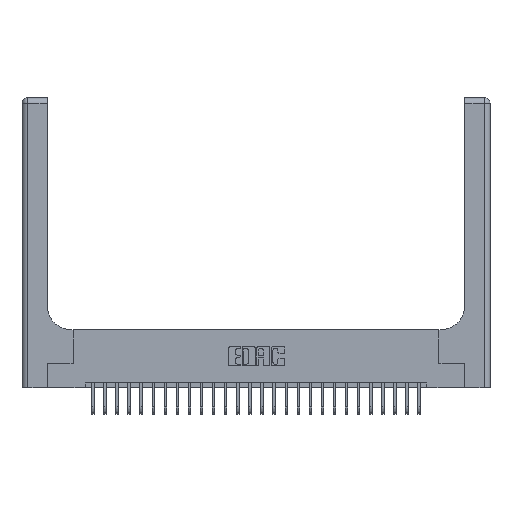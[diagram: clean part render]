
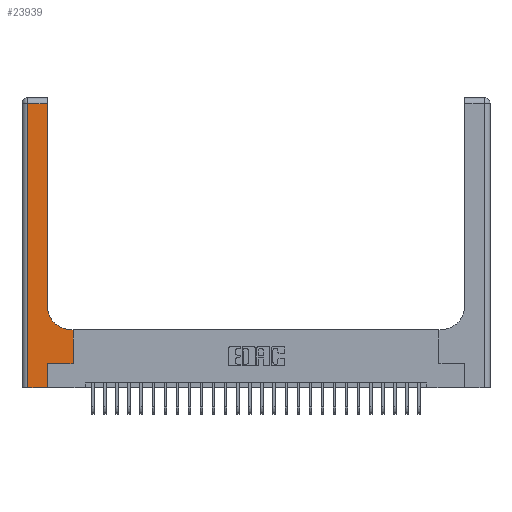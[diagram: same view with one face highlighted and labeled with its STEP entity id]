
A CAD part, top view. The second image highlights one B-rep face of the part: STEP entity #23939.
In plain terms, the highlighted planar face has unit normal (0, 0, 1).
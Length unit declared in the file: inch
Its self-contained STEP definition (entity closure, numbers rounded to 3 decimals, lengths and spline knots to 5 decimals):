
#5 = ORIENTED_EDGE ( 'NONE', *, *, #5332, .T. ) ;
#142 = DIRECTION ( 'NONE',  ( -1., 0., 0. ) ) ;
#563 = CARTESIAN_POINT ( 'NONE',  ( 0.528, 0.25, 0.37 ) ) ;
#609 = VECTOR ( 'NONE', #4721, 39.37008 ) ;
#1825 = CARTESIAN_POINT ( 'NONE',  ( 0.51, 0.6, 0.37 ) ) ;
#2618 = DIRECTION ( 'NONE',  ( 0., 0., -1. ) ) ;
#2772 = DIRECTION ( 'NONE',  ( 0., -1., 0. ) ) ;
#3071 = CIRCLE ( 'NONE', #6296, 0.25 ) ;
#3143 = VERTEX_POINT ( 'NONE', #11806 ) ;
#3183 = AXIS2_PLACEMENT_3D ( 'NONE', #24445, #14598, #14859 ) ;
#3644 = EDGE_LOOP ( 'NONE', ( #12751, #5, #16306, #23933, #14509, #15662, #12771, #17433, #15202 ) ) ;
#4266 = VERTEX_POINT ( 'NONE', #15007 ) ;
#4280 = LINE ( 'NONE', #23768, #8020 ) ;
#4721 = DIRECTION ( 'NONE',  ( -1., 0., 0. ) ) ;
#4760 = DIRECTION ( 'NONE',  ( 1., 0., 0. ) ) ;
#5100 = FACE_OUTER_BOUND ( 'NONE', #3644, .T. ) ;
#5332 = EDGE_CURVE ( 'NONE', #16618, #10583, #10309, .T. ) ;
#5795 = CARTESIAN_POINT ( 'NONE',  ( 0.06, 0., 0.37 ) ) ;
#5812 = CARTESIAN_POINT ( 'NONE',  ( 0.26, 0.6, 0.37 ) ) ;
#5923 = VECTOR ( 'NONE', #142, 39.37008 ) ;
#6296 = AXIS2_PLACEMENT_3D ( 'NONE', #23634, #2618, #4760 ) ;
#6320 = LINE ( 'NONE', #6701, #24600 ) ;
#6701 = CARTESIAN_POINT ( 'NONE',  ( 0.06, 3., 0.37 ) ) ;
#7499 = EDGE_CURVE ( 'NONE', #19654, #24125, #23149, .T. ) ;
#7681 = VECTOR ( 'NONE', #22227, 39.37008 ) ;
#8020 = VECTOR ( 'NONE', #18230, 39.37008 ) ;
#8192 = CARTESIAN_POINT ( 'NONE',  ( 0.26, 2.94, 0.37 ) ) ;
#9288 = PLANE ( 'NONE',  #3183 ) ;
#9572 = EDGE_CURVE ( 'NONE', #4266, #11926, #24064, .T. ) ;
#9664 = VECTOR ( 'NONE', #15995, 39.37008 ) ;
#10309 = LINE ( 'NONE', #23840, #609 ) ;
#10583 = VERTEX_POINT ( 'NONE', #20242 ) ;
#11655 = EDGE_CURVE ( 'NONE', #20416, #16618, #4280, .T. ) ;
#11806 = CARTESIAN_POINT ( 'NONE',  ( 0.528, 0.25, 0.37 ) ) ;
#11926 = VERTEX_POINT ( 'NONE', #19480 ) ;
#12156 = CARTESIAN_POINT ( 'NONE',  ( 0.265, 0.25, 0.37 ) ) ;
#12219 = CARTESIAN_POINT ( 'NONE',  ( 0., 0., 0.37 ) ) ;
#12751 = ORIENTED_EDGE ( 'NONE', *, *, #11655, .T. ) ;
#12771 = ORIENTED_EDGE ( 'NONE', *, *, #23924, .T. ) ;
#14476 = CARTESIAN_POINT ( 'NONE',  ( 0.265, 0., 0.37 ) ) ;
#14509 = ORIENTED_EDGE ( 'NONE', *, *, #9572, .T. ) ;
#14598 = DIRECTION ( 'NONE',  ( 0., 0., -1. ) ) ;
#14759 = EDGE_CURVE ( 'NONE', #20191, #4266, #19942, .T. ) ;
#14859 = DIRECTION ( 'NONE',  ( -1., 0., 0. ) ) ;
#15007 = CARTESIAN_POINT ( 'NONE',  ( 0.265, 0., 0.37 ) ) ;
#15202 = ORIENTED_EDGE ( 'NONE', *, *, #19441, .T. ) ;
#15662 = ORIENTED_EDGE ( 'NONE', *, *, #17805, .T. ) ;
#15995 = DIRECTION ( 'NONE',  ( 0., 1., 0. ) ) ;
#16306 = ORIENTED_EDGE ( 'NONE', *, *, #24664, .T. ) ;
#16618 = VERTEX_POINT ( 'NONE', #8192 ) ;
#17433 = ORIENTED_EDGE ( 'NONE', *, *, #7499, .T. ) ;
#17805 = EDGE_CURVE ( 'NONE', #11926, #3143, #20129, .T. ) ;
#17913 = LINE ( 'NONE', #563, #9664 ) ;
#18230 = DIRECTION ( 'NONE',  ( 0., 1., 0. ) ) ;
#18595 = CARTESIAN_POINT ( 'NONE',  ( 0.528, 0.6, 0.37 ) ) ;
#19303 = VECTOR ( 'NONE', #22205, 39.37008 ) ;
#19441 = EDGE_CURVE ( 'NONE', #24125, #20416, #3071, .T. ) ;
#19480 = CARTESIAN_POINT ( 'NONE',  ( 0.265, 0.25, 0.37 ) ) ;
#19654 = VERTEX_POINT ( 'NONE', #18595 ) ;
#19942 = LINE ( 'NONE', #12219, #7681 ) ;
#20000 = DIRECTION ( 'NONE',  ( 1., 0., 0. ) ) ;
#20129 = LINE ( 'NONE', #12156, #20415 ) ;
#20191 = VERTEX_POINT ( 'NONE', #5795 ) ;
#20242 = CARTESIAN_POINT ( 'NONE',  ( 0.06, 2.94, 0.37 ) ) ;
#20415 = VECTOR ( 'NONE', #20000, 39.37008 ) ;
#20416 = VERTEX_POINT ( 'NONE', #22151 ) ;
#22151 = CARTESIAN_POINT ( 'NONE',  ( 0.26, 0.85, 0.37 ) ) ;
#22205 = DIRECTION ( 'NONE',  ( 0., 1., 0. ) ) ;
#22227 = DIRECTION ( 'NONE',  ( 1., 0., 0. ) ) ;
#23149 = LINE ( 'NONE', #5812, #5923 ) ;
#23634 = CARTESIAN_POINT ( 'NONE',  ( 0.51, 0.85, 0.37 ) ) ;
#23768 = CARTESIAN_POINT ( 'NONE',  ( 0.26, 3., 0.37 ) ) ;
#23840 = CARTESIAN_POINT ( 'NONE',  ( 0., 2.94, 0.37 ) ) ;
#23924 = EDGE_CURVE ( 'NONE', #3143, #19654, #17913, .T. ) ;
#23933 = ORIENTED_EDGE ( 'NONE', *, *, #14759, .T. ) ;
#23939 = ADVANCED_FACE ( 'NONE', ( #5100 ), #9288, .F. ) ;
#24064 = LINE ( 'NONE', #14476, #19303 ) ;
#24125 = VERTEX_POINT ( 'NONE', #1825 ) ;
#24445 = CARTESIAN_POINT ( 'NONE',  ( 0., 3., 0.37 ) ) ;
#24600 = VECTOR ( 'NONE', #2772, 39.37008 ) ;
#24664 = EDGE_CURVE ( 'NONE', #10583, #20191, #6320, .T. ) ;
